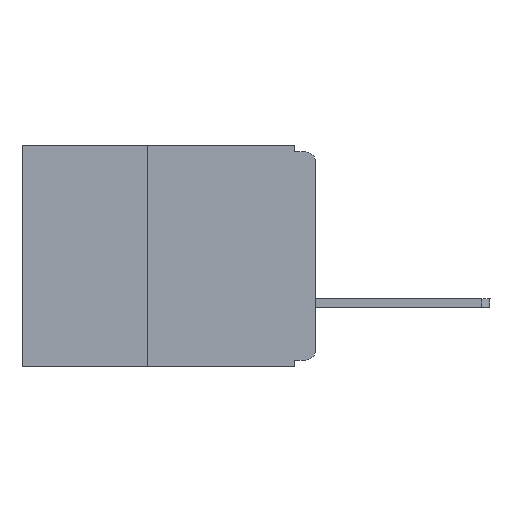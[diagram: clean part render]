
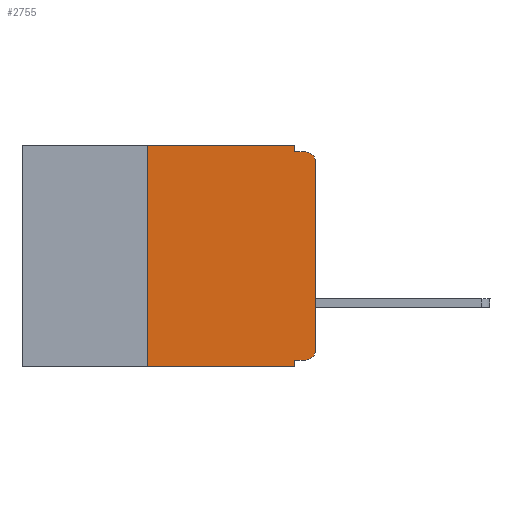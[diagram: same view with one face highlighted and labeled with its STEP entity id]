
A CAD part, left-side view. The second image highlights one B-rep face of the part: STEP entity #2755.
In plain terms, the highlighted planar face has unit normal (-1, 0, 0).
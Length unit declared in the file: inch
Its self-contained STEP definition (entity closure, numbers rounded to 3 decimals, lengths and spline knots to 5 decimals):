
#166 = VERTEX_POINT ( 'NONE', #2141 ) ;
#297 = FACE_OUTER_BOUND ( 'NONE', #9209, .T. ) ;
#615 = ORIENTED_EDGE ( 'NONE', *, *, #3863, .T. ) ;
#625 = CARTESIAN_POINT ( 'NONE',  ( 0., 0., -0.025 ) ) ;
#632 = ORIENTED_EDGE ( 'NONE', *, *, #3220, .T. ) ;
#805 = VECTOR ( 'NONE', #11339, 39.37008 ) ;
#970 = VERTEX_POINT ( 'NONE', #10427 ) ;
#1258 = DIRECTION ( 'NONE',  ( 0., -1., 0. ) ) ;
#1499 = VECTOR ( 'NONE', #6401, 39.37008 ) ;
#1933 = LINE ( 'NONE', #3237, #7014 ) ;
#1954 = LINE ( 'NONE', #4134, #12041 ) ;
#2141 = CARTESIAN_POINT ( 'NONE',  ( 0., 0.031, 0. ) ) ;
#2197 = LINE ( 'NONE', #10832, #4491 ) ;
#2399 = ORIENTED_EDGE ( 'NONE', *, *, #11756, .F. ) ;
#2462 = VERTEX_POINT ( 'NONE', #625 ) ;
#2755 = ADVANCED_FACE ( 'NONE', ( #297 ), #2759, .F. ) ;
#2759 = PLANE ( 'NONE',  #3577 ) ;
#2803 = CARTESIAN_POINT ( 'NONE',  ( 0., 0.015, -0.305 ) ) ;
#2809 = DIRECTION ( 'NONE',  ( 0., 0., -1. ) ) ;
#3061 = EDGE_CURVE ( 'NONE', #4342, #970, #1933, .T. ) ;
#3153 = DIRECTION ( 'NONE',  ( 0., 1., 0. ) ) ;
#3220 = EDGE_CURVE ( 'NONE', #11345, #2462, #12802, .T. ) ;
#3237 = CARTESIAN_POINT ( 'NONE',  ( 0., 0.437, -0.33 ) ) ;
#3317 = DIRECTION ( 'NONE',  ( 0., 0., -1. ) ) ;
#3378 = ORIENTED_EDGE ( 'NONE', *, *, #8802, .F. ) ;
#3422 = CARTESIAN_POINT ( 'NONE',  ( 0., 0.437, 0. ) ) ;
#3460 = VECTOR ( 'NONE', #9684, 39.37008 ) ;
#3514 = LINE ( 'NONE', #5120, #4300 ) ;
#3577 = AXIS2_PLACEMENT_3D ( 'NONE', #3422, #6388, #7623 ) ;
#3652 = CARTESIAN_POINT ( 'NONE',  ( 0., 0.031, -0.01 ) ) ;
#3863 = EDGE_CURVE ( 'NONE', #2462, #4862, #6156, .T. ) ;
#4134 = CARTESIAN_POINT ( 'NONE',  ( 0., 0.031, -0.33 ) ) ;
#4149 = EDGE_CURVE ( 'NONE', #8991, #11345, #9892, .T. ) ;
#4209 = VERTEX_POINT ( 'NONE', #10831 ) ;
#4262 = CARTESIAN_POINT ( 'NONE',  ( 0., 0.437, 0. ) ) ;
#4300 = VECTOR ( 'NONE', #3153, 39.37008 ) ;
#4342 = VERTEX_POINT ( 'NONE', #7390 ) ;
#4491 = VECTOR ( 'NONE', #6955, 39.37008 ) ;
#4616 = CARTESIAN_POINT ( 'NONE',  ( 0., 0., 0. ) ) ;
#4643 = ORIENTED_EDGE ( 'NONE', *, *, #6568, .F. ) ;
#4759 = DIRECTION ( 'NONE',  ( -1., 0., 0. ) ) ;
#4862 = VERTEX_POINT ( 'NONE', #5315 ) ;
#5004 = CARTESIAN_POINT ( 'NONE',  ( 0., 0., -0.305 ) ) ;
#5120 = CARTESIAN_POINT ( 'NONE',  ( 0., 0., -0.32 ) ) ;
#5315 = CARTESIAN_POINT ( 'NONE',  ( 0., 0.015, -0.01 ) ) ;
#5527 = VERTEX_POINT ( 'NONE', #8171 ) ;
#5652 = ORIENTED_EDGE ( 'NONE', *, *, #11567, .F. ) ;
#5937 = ORIENTED_EDGE ( 'NONE', *, *, #3061, .T. ) ;
#6156 = CIRCLE ( 'NONE', #11511, 0.015 ) ;
#6388 = DIRECTION ( 'NONE',  ( 1., 0., 0. ) ) ;
#6401 = DIRECTION ( 'NONE',  ( 0., 0., 1. ) ) ;
#6409 = LINE ( 'NONE', #9679, #8598 ) ;
#6568 = EDGE_CURVE ( 'NONE', #5527, #970, #1954, .T. ) ;
#6773 = ORIENTED_EDGE ( 'NONE', *, *, #8508, .F. ) ;
#6955 = DIRECTION ( 'NONE',  ( 0., -1., 0. ) ) ;
#7014 = VECTOR ( 'NONE', #1258, 39.37008 ) ;
#7226 = ORIENTED_EDGE ( 'NONE', *, *, #10488, .F. ) ;
#7264 = CARTESIAN_POINT ( 'NONE',  ( 0., 0.015, -0.32 ) ) ;
#7390 = CARTESIAN_POINT ( 'NONE',  ( 0., 0.25, -0.33 ) ) ;
#7623 = DIRECTION ( 'NONE',  ( 0., 0., -1. ) ) ;
#7751 = DIRECTION ( 'NONE',  ( 0., 0., -1. ) ) ;
#8171 = CARTESIAN_POINT ( 'NONE',  ( 0., 0.031, -0.32 ) ) ;
#8272 = CARTESIAN_POINT ( 'NONE',  ( 0., 0.25, -0.33 ) ) ;
#8508 = EDGE_CURVE ( 'NONE', #4209, #166, #8834, .T. ) ;
#8598 = VECTOR ( 'NONE', #2809, 39.37008 ) ;
#8802 = EDGE_CURVE ( 'NONE', #9252, #4862, #2197, .T. ) ;
#8834 = LINE ( 'NONE', #4262, #805 ) ;
#8991 = VERTEX_POINT ( 'NONE', #7264 ) ;
#9209 = EDGE_LOOP ( 'NONE', ( #632, #615, #3378, #5652, #6773, #2399, #5937, #4643, #7226, #11562 ) ) ;
#9241 = CARTESIAN_POINT ( 'NONE',  ( 0., 0.015, -0.025 ) ) ;
#9252 = VERTEX_POINT ( 'NONE', #3652 ) ;
#9679 = CARTESIAN_POINT ( 'NONE',  ( 0., 0.031, 0. ) ) ;
#9684 = DIRECTION ( 'NONE',  ( 0., 0., 1. ) ) ;
#9892 = CIRCLE ( 'NONE', #12769, 0.015 ) ;
#10427 = CARTESIAN_POINT ( 'NONE',  ( 0., 0.031, -0.33 ) ) ;
#10488 = EDGE_CURVE ( 'NONE', #8991, #5527, #3514, .T. ) ;
#10831 = CARTESIAN_POINT ( 'NONE',  ( 0., 0.25, 0. ) ) ;
#10832 = CARTESIAN_POINT ( 'NONE',  ( 0., 0., -0.01 ) ) ;
#11205 = DIRECTION ( 'NONE',  ( 0., 0., -1. ) ) ;
#11248 = DIRECTION ( 'NONE',  ( -1., 0., 0. ) ) ;
#11339 = DIRECTION ( 'NONE',  ( 0., -1., 0. ) ) ;
#11345 = VERTEX_POINT ( 'NONE', #5004 ) ;
#11436 = LINE ( 'NONE', #8272, #1499 ) ;
#11511 = AXIS2_PLACEMENT_3D ( 'NONE', #9241, #11248, #11205 ) ;
#11562 = ORIENTED_EDGE ( 'NONE', *, *, #4149, .T. ) ;
#11567 = EDGE_CURVE ( 'NONE', #166, #9252, #6409, .T. ) ;
#11756 = EDGE_CURVE ( 'NONE', #4342, #4209, #11436, .T. ) ;
#12041 = VECTOR ( 'NONE', #3317, 39.37008 ) ;
#12769 = AXIS2_PLACEMENT_3D ( 'NONE', #2803, #4759, #7751 ) ;
#12802 = LINE ( 'NONE', #4616, #3460 ) ;
